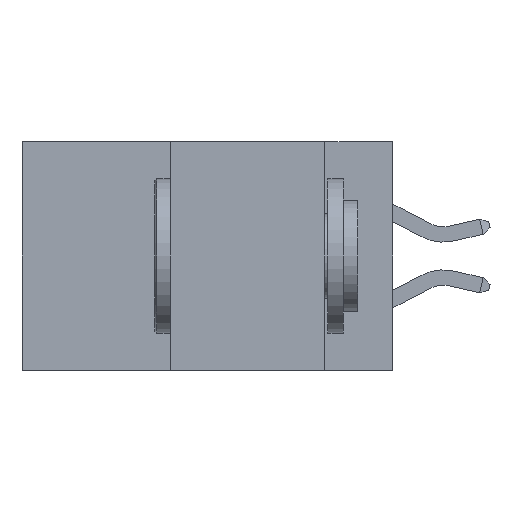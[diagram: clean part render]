
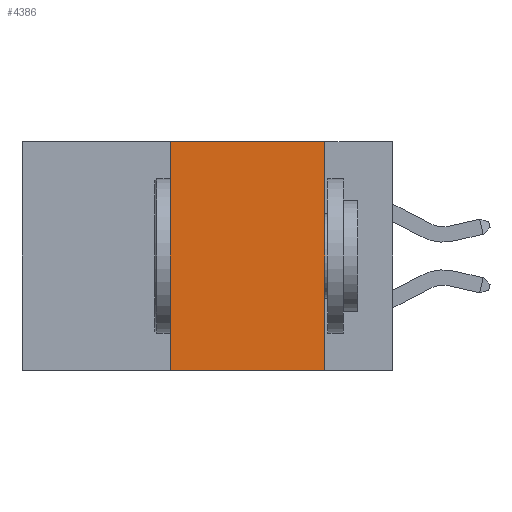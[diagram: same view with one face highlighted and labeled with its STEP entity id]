
A CAD part, left-side view. The second image highlights one B-rep face of the part: STEP entity #4386.
In plain terms, the highlighted planar face has unit normal (-1, 0, 0).
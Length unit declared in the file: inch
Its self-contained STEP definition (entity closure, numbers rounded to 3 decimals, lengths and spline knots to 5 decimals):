
#1264 = ORIENTED_EDGE ( 'NONE', *, *, #14815, .F. ) ;
#2305 = CARTESIAN_POINT ( 'NONE',  ( 0., 0.11, -0.37 ) ) ;
#4386 = ADVANCED_FACE ( 'NONE', ( #6071 ), #39044, .F. ) ;
#6071 = FACE_OUTER_BOUND ( 'NONE', #33617, .T. ) ;
#7692 = DIRECTION ( 'NONE',  ( 1., 0., 0. ) ) ;
#8225 = AXIS2_PLACEMENT_3D ( 'NONE', #29729, #7692, #29590 ) ;
#9695 = ORIENTED_EDGE ( 'NONE', *, *, #27733, .F. ) ;
#9984 = LINE ( 'NONE', #13709, #13395 ) ;
#11285 = CARTESIAN_POINT ( 'NONE',  ( 0., 0.6, -0.37 ) ) ;
#13395 = VECTOR ( 'NONE', #15220, 39.37008 ) ;
#13709 = CARTESIAN_POINT ( 'NONE',  ( 0., 0.36, 0. ) ) ;
#14279 = LINE ( 'NONE', #32899, #38785 ) ;
#14815 = EDGE_CURVE ( 'NONE', #33678, #31435, #9984, .T. ) ;
#15220 = DIRECTION ( 'NONE',  ( 0., 0., 1. ) ) ;
#18221 = CARTESIAN_POINT ( 'NONE',  ( 0., 0.11, 0. ) ) ;
#18886 = CARTESIAN_POINT ( 'NONE',  ( 0., 0.6, 0. ) ) ;
#22027 = DIRECTION ( 'NONE',  ( 0., -1., 0. ) ) ;
#22139 = VECTOR ( 'NONE', #22027, 39.37008 ) ;
#23132 = CARTESIAN_POINT ( 'NONE',  ( 0., 0.36, 0. ) ) ;
#24595 = LINE ( 'NONE', #18886, #22139 ) ;
#26009 = VECTOR ( 'NONE', #30322, 39.37008 ) ;
#26444 = DIRECTION ( 'NONE',  ( 0., 0., -1. ) ) ;
#26638 = VERTEX_POINT ( 'NONE', #2305 ) ;
#27733 = EDGE_CURVE ( 'NONE', #35000, #26638, #14279, .T. ) ;
#29590 = DIRECTION ( 'NONE',  ( 0., 0., -1. ) ) ;
#29729 = CARTESIAN_POINT ( 'NONE',  ( 0., 0.6, 0. ) ) ;
#30311 = ORIENTED_EDGE ( 'NONE', *, *, #39563, .T. ) ;
#30322 = DIRECTION ( 'NONE',  ( 0., -1., 0. ) ) ;
#31435 = VERTEX_POINT ( 'NONE', #23132 ) ;
#32899 = CARTESIAN_POINT ( 'NONE',  ( 0., 0.11, 0. ) ) ;
#33115 = CARTESIAN_POINT ( 'NONE',  ( 0., 0.36, -0.37 ) ) ;
#33175 = EDGE_CURVE ( 'NONE', #31435, #35000, #24595, .T. ) ;
#33617 = EDGE_LOOP ( 'NONE', ( #9695, #39509, #1264, #30311 ) ) ;
#33678 = VERTEX_POINT ( 'NONE', #33115 ) ;
#34360 = LINE ( 'NONE', #11285, #26009 ) ;
#35000 = VERTEX_POINT ( 'NONE', #18221 ) ;
#38785 = VECTOR ( 'NONE', #26444, 39.37008 ) ;
#39044 = PLANE ( 'NONE',  #8225 ) ;
#39509 = ORIENTED_EDGE ( 'NONE', *, *, #33175, .F. ) ;
#39563 = EDGE_CURVE ( 'NONE', #33678, #26638, #34360, .T. ) ;
